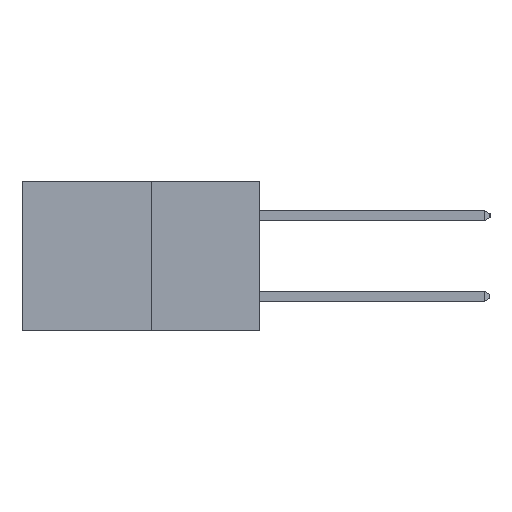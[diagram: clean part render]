
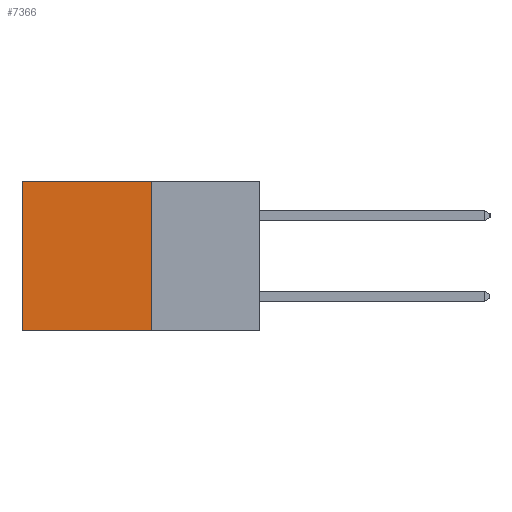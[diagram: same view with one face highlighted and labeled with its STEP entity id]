
A CAD part, left-side view. The second image highlights one B-rep face of the part: STEP entity #7366.
In plain terms, the highlighted planar face has unit normal (-1, 0, 0).
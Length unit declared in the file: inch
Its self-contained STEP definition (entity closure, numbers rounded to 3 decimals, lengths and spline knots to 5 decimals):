
#281 = VERTEX_POINT ( 'NONE', #8869 ) ;
#1003 = LINE ( 'NONE', #2394, #9013 ) ;
#1077 = CARTESIAN_POINT ( 'NONE',  ( 0.277, 0.27, -0.37 ) ) ;
#1221 = VECTOR ( 'NONE', #7185, 39.37008 ) ;
#1604 = CARTESIAN_POINT ( 'NONE',  ( 0.277, 0.27, 0. ) ) ;
#1631 = CARTESIAN_POINT ( 'NONE',  ( 0.277, 0.27, -0.37 ) ) ;
#2071 = ORIENTED_EDGE ( 'NONE', *, *, #9540, .F. ) ;
#2369 = DIRECTION ( 'NONE',  ( 0., 1., 0. ) ) ;
#2394 = CARTESIAN_POINT ( 'NONE',  ( 0.277, 0.59, -0.37 ) ) ;
#2671 = VERTEX_POINT ( 'NONE', #6202 ) ;
#2752 = VERTEX_POINT ( 'NONE', #5430 ) ;
#2936 = ORIENTED_EDGE ( 'NONE', *, *, #7605, .T. ) ;
#3146 = VERTEX_POINT ( 'NONE', #1604 ) ;
#3301 = DIRECTION ( 'NONE',  ( 0., 1., 0. ) ) ;
#3362 = PLANE ( 'NONE',  #3538 ) ;
#3431 = LINE ( 'NONE', #1077, #1221 ) ;
#3538 = AXIS2_PLACEMENT_3D ( 'NONE', #1631, #6578, #4194 ) ;
#3614 = CARTESIAN_POINT ( 'NONE',  ( 0.277, 0.27, -0.37 ) ) ;
#3666 = EDGE_CURVE ( 'NONE', #3146, #2752, #3431, .T. ) ;
#4194 = DIRECTION ( 'NONE',  ( 0., 0., -1. ) ) ;
#4881 = CARTESIAN_POINT ( 'NONE',  ( 0.277, 0.27, 0. ) ) ;
#5021 = ORIENTED_EDGE ( 'NONE', *, *, #3666, .F. ) ;
#5226 = VECTOR ( 'NONE', #3301, 39.37008 ) ;
#5430 = CARTESIAN_POINT ( 'NONE',  ( 0.277, 0.27, -0.37 ) ) ;
#5640 = FACE_OUTER_BOUND ( 'NONE', #7973, .T. ) ;
#6202 = CARTESIAN_POINT ( 'NONE',  ( 0.277, 0.59, 0. ) ) ;
#6335 = EDGE_CURVE ( 'NONE', #3146, #2671, #9260, .T. ) ;
#6578 = DIRECTION ( 'NONE',  ( 1., 0., 0. ) ) ;
#7061 = VECTOR ( 'NONE', #2369, 39.37008 ) ;
#7185 = DIRECTION ( 'NONE',  ( 0., 0., -1. ) ) ;
#7235 = ORIENTED_EDGE ( 'NONE', *, *, #6335, .T. ) ;
#7366 = ADVANCED_FACE ( 'NONE', ( #5640 ), #3362, .F. ) ;
#7462 = LINE ( 'NONE', #3614, #5226 ) ;
#7605 = EDGE_CURVE ( 'NONE', #2671, #281, #1003, .T. ) ;
#7973 = EDGE_LOOP ( 'NONE', ( #2936, #2071, #5021, #7235 ) ) ;
#8869 = CARTESIAN_POINT ( 'NONE',  ( 0.277, 0.59, -0.37 ) ) ;
#9013 = VECTOR ( 'NONE', #9411, 39.37008 ) ;
#9260 = LINE ( 'NONE', #4881, #7061 ) ;
#9411 = DIRECTION ( 'NONE',  ( 0., 0., -1. ) ) ;
#9540 = EDGE_CURVE ( 'NONE', #2752, #281, #7462, .T. ) ;
